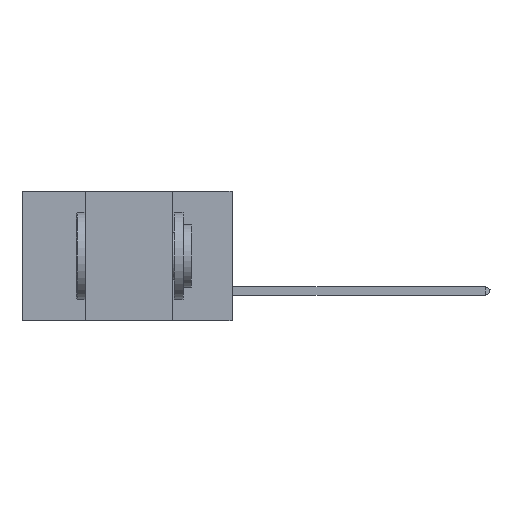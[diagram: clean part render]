
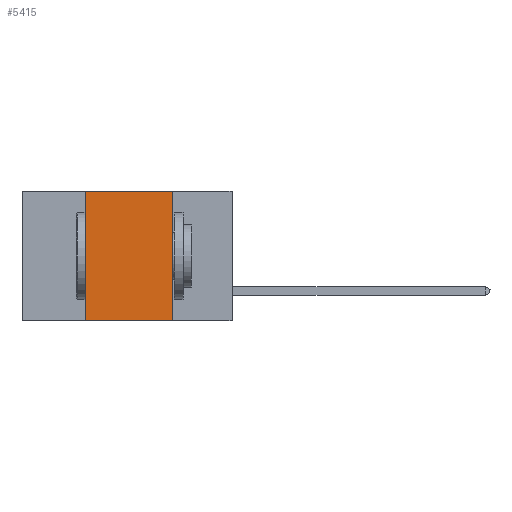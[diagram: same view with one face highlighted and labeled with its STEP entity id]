
A CAD part, left-side view. The second image highlights one B-rep face of the part: STEP entity #5415.
In plain terms, the highlighted planar face has unit normal (-1, 0, 0).
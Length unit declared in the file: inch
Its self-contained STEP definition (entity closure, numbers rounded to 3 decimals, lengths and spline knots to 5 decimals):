
#90 = VERTEX_POINT ( 'NONE', #47982 ) ;
#2361 = DIRECTION ( 'NONE',  ( 0., 0., -1. ) ) ;
#5415 = ADVANCED_FACE ( 'NONE', ( #12369 ), #12613, .F. ) ;
#5670 = ORIENTED_EDGE ( 'NONE', *, *, #49043, .F. ) ;
#11902 = DIRECTION ( 'NONE',  ( 0., 0., 1. ) ) ;
#12062 = CARTESIAN_POINT ( 'NONE',  ( 0., 0.42, 0. ) ) ;
#12369 = FACE_OUTER_BOUND ( 'NONE', #41824, .T. ) ;
#12613 = PLANE ( 'NONE',  #31926 ) ;
#13311 = EDGE_CURVE ( 'NONE', #13618, #32685, #24887, .T. ) ;
#13390 = VECTOR ( 'NONE', #20836, 39.37008 ) ;
#13618 = VERTEX_POINT ( 'NONE', #48758 ) ;
#14914 = LINE ( 'NONE', #25595, #23909 ) ;
#15638 = VECTOR ( 'NONE', #11902, 39.37008 ) ;
#19917 = DIRECTION ( 'NONE',  ( 0., -1., 0. ) ) ;
#20836 = DIRECTION ( 'NONE',  ( 0., -1., 0. ) ) ;
#21378 = VERTEX_POINT ( 'NONE', #45190 ) ;
#23909 = VECTOR ( 'NONE', #2361, 39.37008 ) ;
#24887 = LINE ( 'NONE', #39169, #34134 ) ;
#25595 = CARTESIAN_POINT ( 'NONE',  ( 0., 0.17, 0. ) ) ;
#26260 = ORIENTED_EDGE ( 'NONE', *, *, #40078, .F. ) ;
#29953 = ORIENTED_EDGE ( 'NONE', *, *, #33250, .T. ) ;
#31926 = AXIS2_PLACEMENT_3D ( 'NONE', #35904, #39811, #47319 ) ;
#32685 = VERTEX_POINT ( 'NONE', #41356 ) ;
#33250 = EDGE_CURVE ( 'NONE', #21378, #90, #40739, .T. ) ;
#34134 = VECTOR ( 'NONE', #19917, 39.37008 ) ;
#35904 = CARTESIAN_POINT ( 'NONE',  ( 0., 0.6, 0. ) ) ;
#39169 = CARTESIAN_POINT ( 'NONE',  ( 0., 0.6, 0. ) ) ;
#39811 = DIRECTION ( 'NONE',  ( 1., 0., 0. ) ) ;
#40078 = EDGE_CURVE ( 'NONE', #21378, #13618, #40535, .T. ) ;
#40535 = LINE ( 'NONE', #12062, #15638 ) ;
#40739 = LINE ( 'NONE', #48268, #13390 ) ;
#41356 = CARTESIAN_POINT ( 'NONE',  ( 0., 0.17, 0. ) ) ;
#41824 = EDGE_LOOP ( 'NONE', ( #5670, #47366, #26260, #29953 ) ) ;
#45190 = CARTESIAN_POINT ( 'NONE',  ( 0., 0.42, -0.37 ) ) ;
#47319 = DIRECTION ( 'NONE',  ( 0., 0., -1. ) ) ;
#47366 = ORIENTED_EDGE ( 'NONE', *, *, #13311, .F. ) ;
#47982 = CARTESIAN_POINT ( 'NONE',  ( 0., 0.17, -0.37 ) ) ;
#48268 = CARTESIAN_POINT ( 'NONE',  ( 0., 0.6, -0.37 ) ) ;
#48758 = CARTESIAN_POINT ( 'NONE',  ( 0., 0.42, 0. ) ) ;
#49043 = EDGE_CURVE ( 'NONE', #32685, #90, #14914, .T. ) ;
